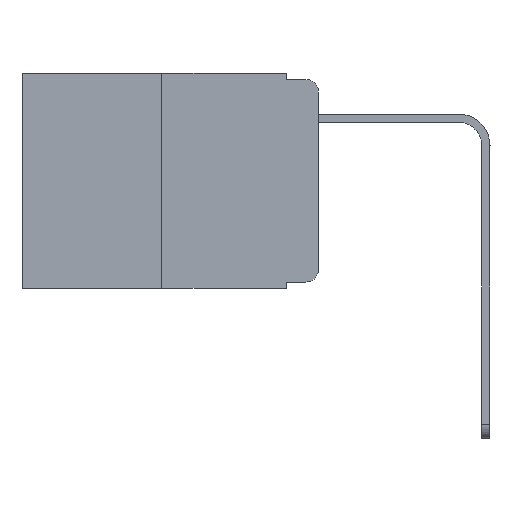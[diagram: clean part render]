
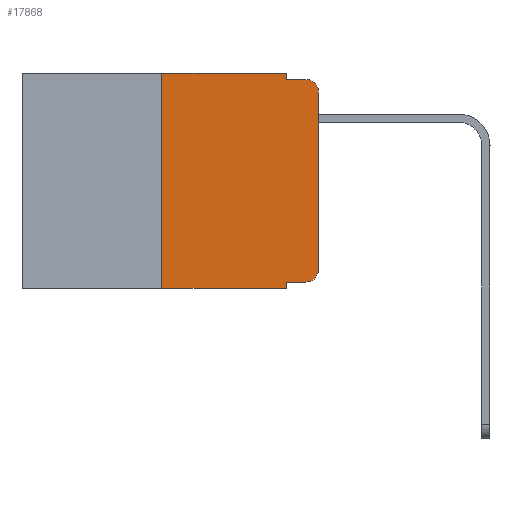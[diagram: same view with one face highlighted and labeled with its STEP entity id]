
A CAD part, left-side view. The second image highlights one B-rep face of the part: STEP entity #17868.
In plain terms, the highlighted planar face has unit normal (-1, 0, 0).
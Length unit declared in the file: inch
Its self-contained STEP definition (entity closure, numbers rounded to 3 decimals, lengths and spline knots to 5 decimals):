
#36 = VERTEX_POINT ( 'NONE', #1681 ) ;
#693 = DIRECTION ( 'NONE',  ( -1., 0., 0. ) ) ;
#921 = CARTESIAN_POINT ( 'NONE',  ( 0., 0.25, -0.343 ) ) ;
#1106 = DIRECTION ( 'NONE',  ( 0., -1., 0. ) ) ;
#1236 = VERTEX_POINT ( 'NONE', #13550 ) ;
#1262 = VERTEX_POINT ( 'NONE', #10586 ) ;
#1416 = VERTEX_POINT ( 'NONE', #16202 ) ;
#1681 = CARTESIAN_POINT ( 'NONE',  ( 0., 0., -0.313 ) ) ;
#1752 = CIRCLE ( 'NONE', #10407, 0.02 ) ;
#1892 = EDGE_CURVE ( 'NONE', #14623, #1416, #7436, .T. ) ;
#1935 = VERTEX_POINT ( 'NONE', #11791 ) ;
#1941 = EDGE_CURVE ( 'NONE', #1935, #13576, #10239, .T. ) ;
#2597 = ORIENTED_EDGE ( 'NONE', *, *, #1941, .F. ) ;
#2609 = ORIENTED_EDGE ( 'NONE', *, *, #4792, .T. ) ;
#3104 = ORIENTED_EDGE ( 'NONE', *, *, #3281, .F. ) ;
#3117 = DIRECTION ( 'NONE',  ( 0., -1., 0. ) ) ;
#3207 = EDGE_CURVE ( 'NONE', #17331, #36, #1752, .T. ) ;
#3281 = EDGE_CURVE ( 'NONE', #8799, #1935, #18701, .T. ) ;
#3314 = EDGE_CURVE ( 'NONE', #11243, #1416, #12943, .T. ) ;
#3968 = ORIENTED_EDGE ( 'NONE', *, *, #14598, .T. ) ;
#4071 = CARTESIAN_POINT ( 'NONE',  ( 0., 0.051, 0. ) ) ;
#4153 = DIRECTION ( 'NONE',  ( 0., 0., -1. ) ) ;
#4221 = CARTESIAN_POINT ( 'NONE',  ( 0., 0.473, 0. ) ) ;
#4457 = CARTESIAN_POINT ( 'NONE',  ( 0., 0.051, 0. ) ) ;
#4792 = EDGE_CURVE ( 'NONE', #1262, #13576, #14299, .T. ) ;
#5049 = FACE_OUTER_BOUND ( 'NONE', #12044, .T. ) ;
#5368 = VECTOR ( 'NONE', #9978, 39.37008 ) ;
#5419 = DIRECTION ( 'NONE',  ( -1., 0., 0. ) ) ;
#6311 = VECTOR ( 'NONE', #16281, 39.37008 ) ;
#6517 = LINE ( 'NONE', #8085, #18037 ) ;
#6860 = ORIENTED_EDGE ( 'NONE', *, *, #3314, .F. ) ;
#7244 = CARTESIAN_POINT ( 'NONE',  ( 0., 0.051, 0. ) ) ;
#7378 = VECTOR ( 'NONE', #3117, 39.37008 ) ;
#7436 = LINE ( 'NONE', #17587, #12529 ) ;
#7549 = LINE ( 'NONE', #14496, #15190 ) ;
#8085 = CARTESIAN_POINT ( 'NONE',  ( 0., 0., 0. ) ) ;
#8393 = PLANE ( 'NONE',  #15371 ) ;
#8799 = VERTEX_POINT ( 'NONE', #4457 ) ;
#9641 = DIRECTION ( 'NONE',  ( 0., 0., 1. ) ) ;
#9978 = DIRECTION ( 'NONE',  ( 0., 0., -1. ) ) ;
#10232 = LINE ( 'NONE', #15624, #10931 ) ;
#10239 = LINE ( 'NONE', #16212, #6311 ) ;
#10350 = EDGE_CURVE ( 'NONE', #14623, #1236, #7549, .T. ) ;
#10407 = AXIS2_PLACEMENT_3D ( 'NONE', #18600, #5419, #11060 ) ;
#10586 = CARTESIAN_POINT ( 'NONE',  ( 0., 0., -0.03 ) ) ;
#10931 = VECTOR ( 'NONE', #1106, 39.37008 ) ;
#11036 = AXIS2_PLACEMENT_3D ( 'NONE', #18213, #693, #13834 ) ;
#11060 = DIRECTION ( 'NONE',  ( 0., 0., -1. ) ) ;
#11141 = ORIENTED_EDGE ( 'NONE', *, *, #10350, .F. ) ;
#11243 = VERTEX_POINT ( 'NONE', #14412 ) ;
#11365 = DIRECTION ( 'NONE',  ( 1., 0., 0. ) ) ;
#11754 = CARTESIAN_POINT ( 'NONE',  ( 0., 0.02, -0.333 ) ) ;
#11791 = CARTESIAN_POINT ( 'NONE',  ( 0., 0.051, -0.01 ) ) ;
#12044 = EDGE_LOOP ( 'NONE', ( #3968, #2609, #2597, #3104, #18281, #11141, #16270, #6860, #17935, #15082 ) ) ;
#12529 = VECTOR ( 'NONE', #14447, 39.37008 ) ;
#12891 = DIRECTION ( 'NONE',  ( 0., 0., 1. ) ) ;
#12943 = LINE ( 'NONE', #7244, #16862 ) ;
#13550 = CARTESIAN_POINT ( 'NONE',  ( 0., 0.25, 0. ) ) ;
#13576 = VERTEX_POINT ( 'NONE', #14012 ) ;
#13711 = EDGE_CURVE ( 'NONE', #11243, #17331, #10232, .T. ) ;
#13834 = DIRECTION ( 'NONE',  ( 0., 0., -1. ) ) ;
#14012 = CARTESIAN_POINT ( 'NONE',  ( 0., 0.02, -0.01 ) ) ;
#14299 = CIRCLE ( 'NONE', #11036, 0.02 ) ;
#14354 = DIRECTION ( 'NONE',  ( 0., 0., -1. ) ) ;
#14412 = CARTESIAN_POINT ( 'NONE',  ( 0., 0.051, -0.333 ) ) ;
#14447 = DIRECTION ( 'NONE',  ( 0., -1., 0. ) ) ;
#14496 = CARTESIAN_POINT ( 'NONE',  ( 0., 0.25, 0. ) ) ;
#14598 = EDGE_CURVE ( 'NONE', #36, #1262, #6517, .T. ) ;
#14623 = VERTEX_POINT ( 'NONE', #921 ) ;
#15082 = ORIENTED_EDGE ( 'NONE', *, *, #3207, .T. ) ;
#15190 = VECTOR ( 'NONE', #12891, 39.37008 ) ;
#15371 = AXIS2_PLACEMENT_3D ( 'NONE', #4221, #11365, #4153 ) ;
#15466 = LINE ( 'NONE', #17690, #7378 ) ;
#15624 = CARTESIAN_POINT ( 'NONE',  ( 0., 0.051, -0.333 ) ) ;
#16190 = EDGE_CURVE ( 'NONE', #1236, #8799, #15466, .T. ) ;
#16202 = CARTESIAN_POINT ( 'NONE',  ( 0., 0.051, -0.343 ) ) ;
#16212 = CARTESIAN_POINT ( 'NONE',  ( 0., 0.051, -0.01 ) ) ;
#16270 = ORIENTED_EDGE ( 'NONE', *, *, #1892, .T. ) ;
#16281 = DIRECTION ( 'NONE',  ( 0., -1., 0. ) ) ;
#16862 = VECTOR ( 'NONE', #14354, 39.37008 ) ;
#17331 = VERTEX_POINT ( 'NONE', #11754 ) ;
#17587 = CARTESIAN_POINT ( 'NONE',  ( 0., 0.473, -0.343 ) ) ;
#17690 = CARTESIAN_POINT ( 'NONE',  ( 0., 0.473, 0. ) ) ;
#17868 = ADVANCED_FACE ( 'NONE', ( #5049 ), #8393, .F. ) ;
#17935 = ORIENTED_EDGE ( 'NONE', *, *, #13711, .T. ) ;
#18037 = VECTOR ( 'NONE', #9641, 39.37008 ) ;
#18213 = CARTESIAN_POINT ( 'NONE',  ( 0., 0.02, -0.03 ) ) ;
#18281 = ORIENTED_EDGE ( 'NONE', *, *, #16190, .F. ) ;
#18600 = CARTESIAN_POINT ( 'NONE',  ( 0., 0.02, -0.313 ) ) ;
#18701 = LINE ( 'NONE', #4071, #5368 ) ;
